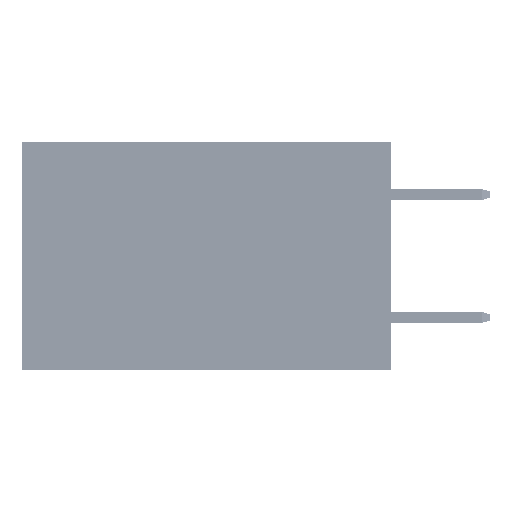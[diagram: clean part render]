
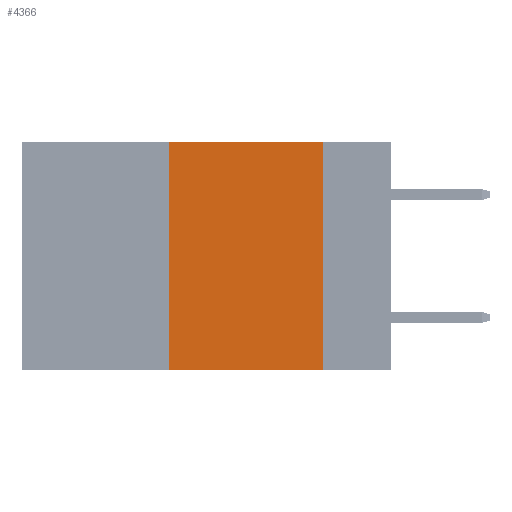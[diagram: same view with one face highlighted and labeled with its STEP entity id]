
A CAD part, left-side view. The second image highlights one B-rep face of the part: STEP entity #4366.
In plain terms, the highlighted planar face has unit normal (-1, 0, 0).
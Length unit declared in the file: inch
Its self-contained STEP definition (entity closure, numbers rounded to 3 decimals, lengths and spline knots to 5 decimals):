
#160 = EDGE_LOOP ( 'NONE', ( #4547, #10757, #2397, #51529 ) ) ;
#279 = CARTESIAN_POINT ( 'NONE',  ( 0., 0.6, 0. ) ) ;
#790 = CARTESIAN_POINT ( 'NONE',  ( 0., 0.11, 0. ) ) ;
#2397 = ORIENTED_EDGE ( 'NONE', *, *, #17517, .F. ) ;
#3999 = DIRECTION ( 'NONE',  ( 0., -1., 0. ) ) ;
#4366 = ADVANCED_FACE ( 'NONE', ( #19471 ), #20644, .F. ) ;
#4547 = ORIENTED_EDGE ( 'NONE', *, *, #11048, .F. ) ;
#8681 = LINE ( 'NONE', #51485, #29066 ) ;
#8752 = VECTOR ( 'NONE', #3999, 39.37008 ) ;
#10161 = VERTEX_POINT ( 'NONE', #790 ) ;
#10757 = ORIENTED_EDGE ( 'NONE', *, *, #45084, .F. ) ;
#11048 = EDGE_CURVE ( 'NONE', #10161, #16506, #8681, .T. ) ;
#12654 = DIRECTION ( 'NONE',  ( 0., 0., -1. ) ) ;
#12657 = VERTEX_POINT ( 'NONE', #39548 ) ;
#15791 = EDGE_CURVE ( 'NONE', #24703, #16506, #47380, .T. ) ;
#16506 = VERTEX_POINT ( 'NONE', #19450 ) ;
#17517 = EDGE_CURVE ( 'NONE', #24703, #12657, #37222, .T. ) ;
#19450 = CARTESIAN_POINT ( 'NONE',  ( 0., 0.11, -0.37 ) ) ;
#19471 = FACE_OUTER_BOUND ( 'NONE', #160, .T. ) ;
#20644 = PLANE ( 'NONE',  #29228 ) ;
#24472 = DIRECTION ( 'NONE',  ( 0., 0., 1. ) ) ;
#24703 = VERTEX_POINT ( 'NONE', #30012 ) ;
#27352 = CARTESIAN_POINT ( 'NONE',  ( 0., 0.6, -0.37 ) ) ;
#29066 = VECTOR ( 'NONE', #47615, 39.37008 ) ;
#29228 = AXIS2_PLACEMENT_3D ( 'NONE', #279, #37024, #12654 ) ;
#30012 = CARTESIAN_POINT ( 'NONE',  ( 0., 0.36, -0.37 ) ) ;
#30417 = LINE ( 'NONE', #44529, #8752 ) ;
#35930 = VECTOR ( 'NONE', #24472, 39.37008 ) ;
#37024 = DIRECTION ( 'NONE',  ( 1., 0., 0. ) ) ;
#37222 = LINE ( 'NONE', #40607, #35930 ) ;
#39548 = CARTESIAN_POINT ( 'NONE',  ( 0., 0.36, 0. ) ) ;
#40607 = CARTESIAN_POINT ( 'NONE',  ( 0., 0.36, 0. ) ) ;
#44529 = CARTESIAN_POINT ( 'NONE',  ( 0., 0.6, 0. ) ) ;
#45084 = EDGE_CURVE ( 'NONE', #12657, #10161, #30417, .T. ) ;
#46114 = VECTOR ( 'NONE', #47491, 39.37008 ) ;
#47380 = LINE ( 'NONE', #27352, #46114 ) ;
#47491 = DIRECTION ( 'NONE',  ( 0., -1., 0. ) ) ;
#47615 = DIRECTION ( 'NONE',  ( 0., 0., -1. ) ) ;
#51485 = CARTESIAN_POINT ( 'NONE',  ( 0., 0.11, 0. ) ) ;
#51529 = ORIENTED_EDGE ( 'NONE', *, *, #15791, .T. ) ;
